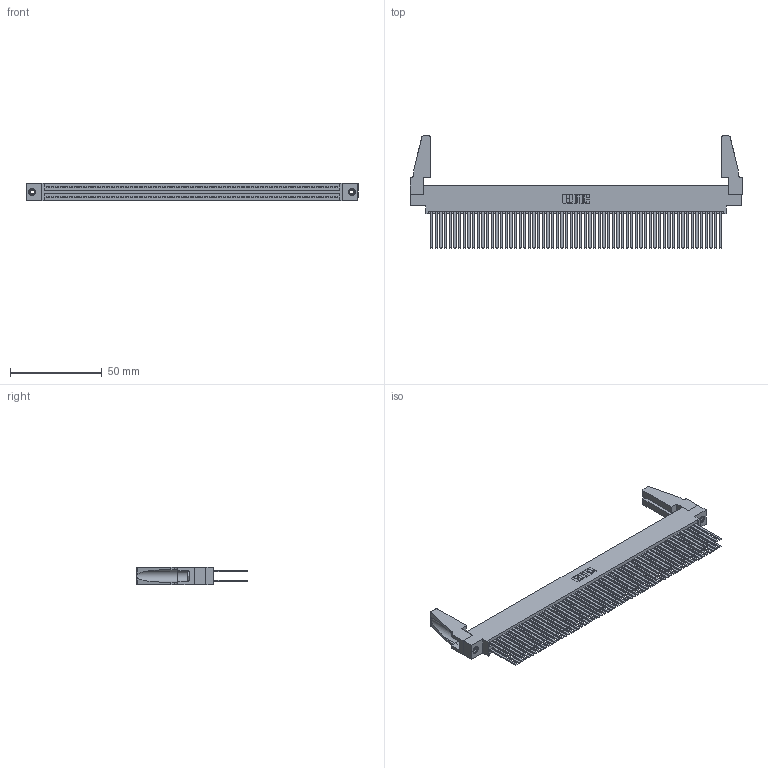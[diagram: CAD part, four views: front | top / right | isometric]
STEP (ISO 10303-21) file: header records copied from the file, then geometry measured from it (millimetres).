
FILE_DESCRIPTION (( 'STEP AP203' ), '1' );
FILE_NAME ('395-126-544-888.STEP', '2019-10-28T15:57:44', ( '' ), ( '' ), 'SwSTEP 2.0', 'SolidWorks 2016', '' );
FILE_SCHEMA (( 'CONFIG_CONTROL_DESIGN' ));
Length unit declared in the file: inch
Products named in the file (5): 345-292-001_345-293-144; 345-250-001_345-250-001-102; 345-220-078_345-220-088; 395-126-544-888; 345 Part_0.170 Offset - 0.156 Dia-TH
Assembly tree (131 placements, depth 2):
  395-126-544-888
    345 Part_0.170 Offset - 0.156 Dia-TH
    345-292-001_345-293-144  x126
    345-250-001_345-250-001-102  x2
    345-220-078_345-220-088  x2
Bounding box: 181.25 x 61.14 x 9.4 mm (x, y, z)
Volume: 22707.5 mm3; surface area: 37607 mm2
Topology: 131 solids, 131 shells, 5798 faces, 17173 edges, 11270 vertices
Faces by surface type: plane 3810, cylinder 1972, cone 12, torus 4
Entity records: 48700 total; most frequent: CARTESIAN_POINT 8138, ORIENTED_EDGE 8032, DIRECTION 7152, EDGE_CURVE 4016, LINE 3594, VECTOR 3594, VERTEX_POINT 2670, AXIS2_PLACEMENT_3D 1779
